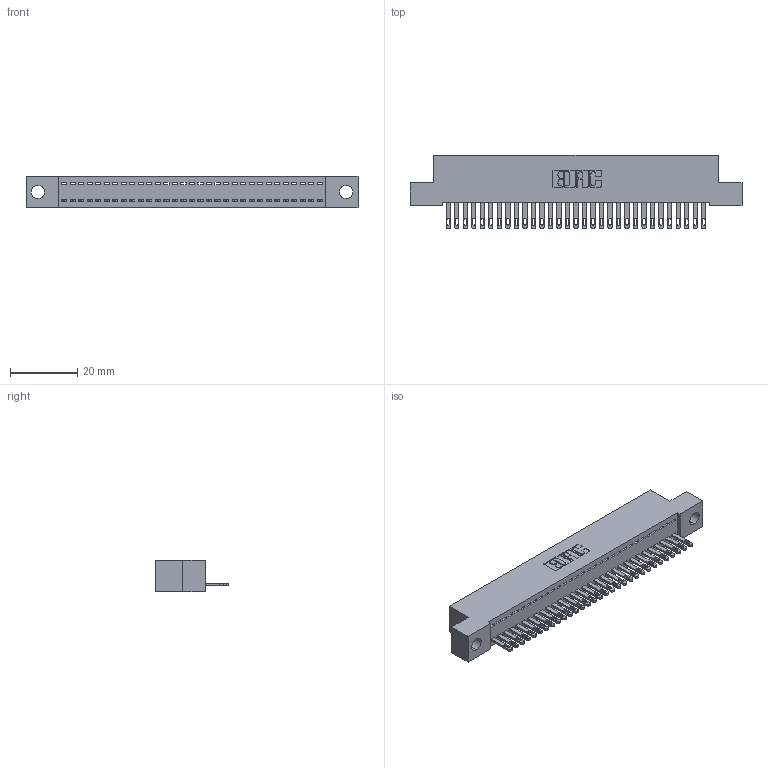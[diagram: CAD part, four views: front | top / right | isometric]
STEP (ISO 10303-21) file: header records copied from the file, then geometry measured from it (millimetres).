
FILE_DESCRIPTION (( 'STEP AP203' ), '1' );
FILE_NAME ('342-031-500-104.STEP', '2019-10-02T05:19:16', ( '' ), ( '' ), 'SwSTEP 2.0', 'SolidWorks 2016', '' );
FILE_SCHEMA (( 'CONFIG_CONTROL_DESIGN' ));
Length unit declared in the file: inch
Products named in the file (3): 342 Part_.156 TH; 345-292-001_345-293-100; 342-031-500-104
Assembly tree (32 placements, depth 2):
  342-031-500-104
    342 Part_.156 TH
    345-292-001_345-293-100  x31
Bounding box: 99.06 x 21.85 x 9.4 mm (x, y, z)
Volume: 8577.2 mm3; surface area: 12269.7 mm2
Topology: 32 solids, 32 shells, 1784 faces, 5507 edges, 3670 vertices
Faces by surface type: plane 1182, cylinder 602
Entity records: 20175 total; most frequent: CARTESIAN_POINT 3487, ORIENTED_EDGE 3454, DIRECTION 2965, EDGE_CURVE 1727, LINE 1595, VECTOR 1595, VERTEX_POINT 1150, AXIS2_PLACEMENT_3D 685
